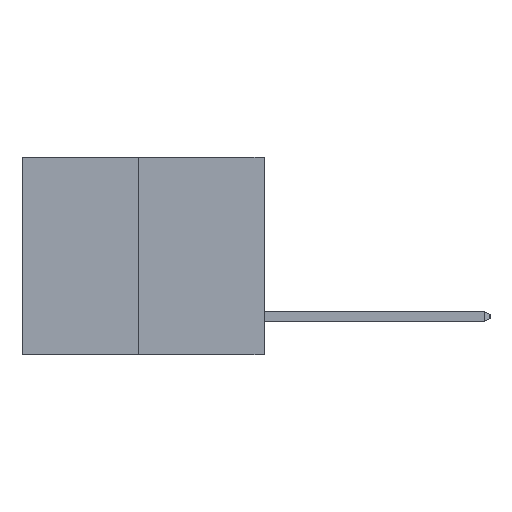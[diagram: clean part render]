
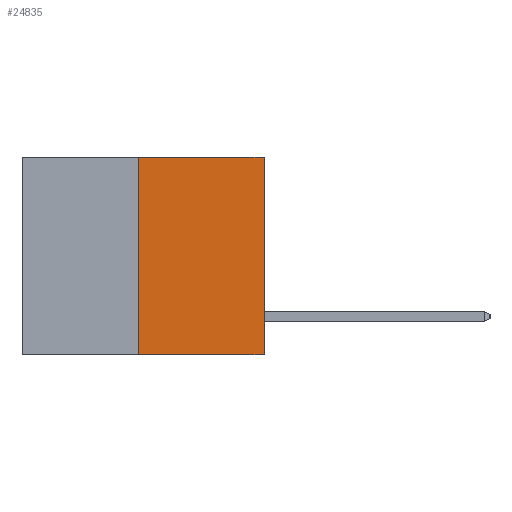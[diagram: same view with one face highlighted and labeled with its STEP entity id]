
A CAD part, left-side view. The second image highlights one B-rep face of the part: STEP entity #24835.
In plain terms, the highlighted planar face has unit normal (-1, 0, 0).
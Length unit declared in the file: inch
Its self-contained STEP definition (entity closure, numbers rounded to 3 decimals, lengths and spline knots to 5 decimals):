
#2082 = ORIENTED_EDGE ( 'NONE', *, *, #16080, .F. ) ;
#2219 = CARTESIAN_POINT ( 'NONE',  ( 0., 0., 0. ) ) ;
#2412 = DIRECTION ( 'NONE',  ( 0., 0., 1. ) ) ;
#2416 = CARTESIAN_POINT ( 'NONE',  ( 0., 0.312, -0.49 ) ) ;
#2843 = PLANE ( 'NONE',  #23358 ) ;
#3118 = LINE ( 'NONE', #15870, #4515 ) ;
#3698 = VERTEX_POINT ( 'NONE', #4677 ) ;
#3785 = EDGE_CURVE ( 'NONE', #15115, #3698, #19549, .T. ) ;
#4515 = VECTOR ( 'NONE', #2412, 39.37008 ) ;
#4677 = CARTESIAN_POINT ( 'NONE',  ( 0., 0., -0.49 ) ) ;
#5350 = DIRECTION ( 'NONE',  ( 0., 0., -1. ) ) ;
#5528 = EDGE_CURVE ( 'NONE', #15115, #9663, #3118, .T. ) ;
#5599 = DIRECTION ( 'NONE',  ( 0., 0., 1. ) ) ;
#6525 = LINE ( 'NONE', #7209, #21869 ) ;
#7209 = CARTESIAN_POINT ( 'NONE',  ( 0., 0.6, 0. ) ) ;
#7492 = CARTESIAN_POINT ( 'NONE',  ( 0., 0.6, 0. ) ) ;
#7708 = DIRECTION ( 'NONE',  ( 1., 0., 0. ) ) ;
#9663 = VERTEX_POINT ( 'NONE', #24267 ) ;
#9877 = FACE_OUTER_BOUND ( 'NONE', #28760, .T. ) ;
#10391 = EDGE_CURVE ( 'NONE', #3698, #25221, #24531, .T. ) ;
#15115 = VERTEX_POINT ( 'NONE', #2416 ) ;
#15870 = CARTESIAN_POINT ( 'NONE',  ( 0., 0.312, -0.49 ) ) ;
#16080 = EDGE_CURVE ( 'NONE', #9663, #25221, #6525, .T. ) ;
#18267 = CARTESIAN_POINT ( 'NONE',  ( 0., 0., 0. ) ) ;
#18318 = DIRECTION ( 'NONE',  ( 0., -1., 0. ) ) ;
#18406 = CARTESIAN_POINT ( 'NONE',  ( 0., 0.6, -0.49 ) ) ;
#19549 = LINE ( 'NONE', #18406, #28573 ) ;
#21275 = ORIENTED_EDGE ( 'NONE', *, *, #5528, .F. ) ;
#21762 = VECTOR ( 'NONE', #5599, 39.37008 ) ;
#21869 = VECTOR ( 'NONE', #22790, 39.37008 ) ;
#22790 = DIRECTION ( 'NONE',  ( 0., -1., 0. ) ) ;
#23358 = AXIS2_PLACEMENT_3D ( 'NONE', #7492, #7708, #5350 ) ;
#24066 = ORIENTED_EDGE ( 'NONE', *, *, #10391, .T. ) ;
#24267 = CARTESIAN_POINT ( 'NONE',  ( 0., 0.312, 0. ) ) ;
#24531 = LINE ( 'NONE', #18267, #21762 ) ;
#24728 = ORIENTED_EDGE ( 'NONE', *, *, #3785, .T. ) ;
#24835 = ADVANCED_FACE ( 'NONE', ( #9877 ), #2843, .F. ) ;
#25221 = VERTEX_POINT ( 'NONE', #2219 ) ;
#28573 = VECTOR ( 'NONE', #18318, 39.37008 ) ;
#28760 = EDGE_LOOP ( 'NONE', ( #21275, #24728, #24066, #2082 ) ) ;
